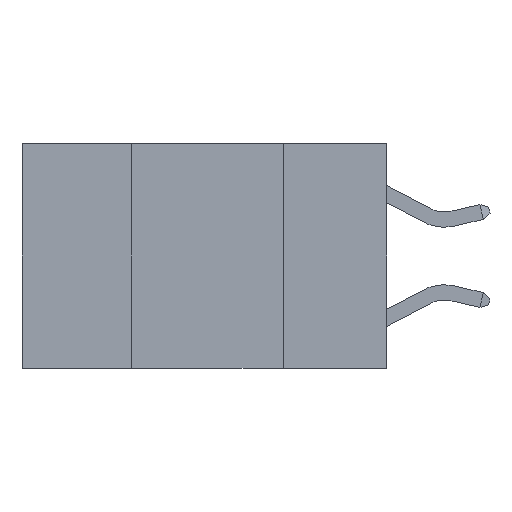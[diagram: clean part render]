
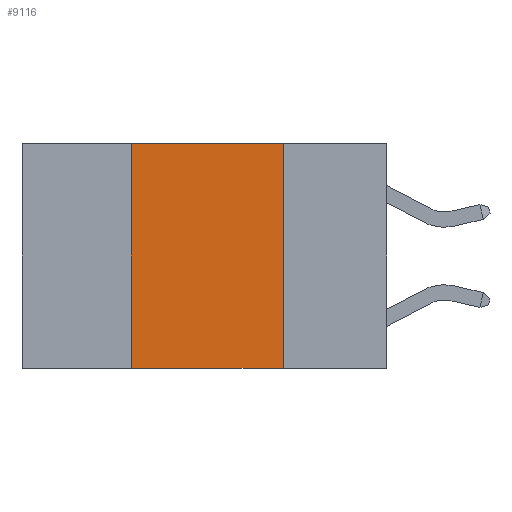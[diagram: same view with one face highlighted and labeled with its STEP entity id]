
A CAD part, left-side view. The second image highlights one B-rep face of the part: STEP entity #9116.
In plain terms, the highlighted planar face has unit normal (-1, 0, 0).
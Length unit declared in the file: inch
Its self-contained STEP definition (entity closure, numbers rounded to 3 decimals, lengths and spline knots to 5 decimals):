
#62 = VECTOR ( 'NONE', #11894, 39.37008 ) ;
#126 = CARTESIAN_POINT ( 'NONE',  ( 0., 0.17, -0.37 ) ) ;
#398 = EDGE_LOOP ( 'NONE', ( #6919, #1309, #10537, #2704 ) ) ;
#486 = VERTEX_POINT ( 'NONE', #126 ) ;
#876 = EDGE_CURVE ( 'NONE', #2681, #11668, #10530, .T. ) ;
#1148 = VECTOR ( 'NONE', #3684, 39.37008 ) ;
#1309 = ORIENTED_EDGE ( 'NONE', *, *, #13399, .F. ) ;
#2628 = LINE ( 'NONE', #9299, #4996 ) ;
#2681 = VERTEX_POINT ( 'NONE', #8434 ) ;
#2704 = ORIENTED_EDGE ( 'NONE', *, *, #11285, .T. ) ;
#3471 = DIRECTION ( 'NONE',  ( 0., 0., -1. ) ) ;
#3684 = DIRECTION ( 'NONE',  ( 0., -1., 0. ) ) ;
#4273 = CARTESIAN_POINT ( 'NONE',  ( 0., 0.17, 0. ) ) ;
#4996 = VECTOR ( 'NONE', #13877, 39.37008 ) ;
#6803 = PLANE ( 'NONE',  #7545 ) ;
#6822 = CARTESIAN_POINT ( 'NONE',  ( 0., 0.42, 0. ) ) ;
#6919 = ORIENTED_EDGE ( 'NONE', *, *, #10854, .F. ) ;
#7545 = AXIS2_PLACEMENT_3D ( 'NONE', #12343, #10077, #3471 ) ;
#7910 = VECTOR ( 'NONE', #11488, 39.37008 ) ;
#8055 = CARTESIAN_POINT ( 'NONE',  ( 0., 0.6, 0. ) ) ;
#8434 = CARTESIAN_POINT ( 'NONE',  ( 0., 0.42, -0.37 ) ) ;
#8445 = CARTESIAN_POINT ( 'NONE',  ( 0., 0.17, 0. ) ) ;
#9116 = ADVANCED_FACE ( 'NONE', ( #13704 ), #6803, .F. ) ;
#9299 = CARTESIAN_POINT ( 'NONE',  ( 0., 0.6, -0.37 ) ) ;
#9623 = VERTEX_POINT ( 'NONE', #4273 ) ;
#9991 = LINE ( 'NONE', #8055, #1148 ) ;
#10077 = DIRECTION ( 'NONE',  ( 1., 0., 0. ) ) ;
#10307 = LINE ( 'NONE', #8445, #62 ) ;
#10530 = LINE ( 'NONE', #12134, #7910 ) ;
#10537 = ORIENTED_EDGE ( 'NONE', *, *, #876, .F. ) ;
#10854 = EDGE_CURVE ( 'NONE', #9623, #486, #10307, .T. ) ;
#11285 = EDGE_CURVE ( 'NONE', #2681, #486, #2628, .T. ) ;
#11488 = DIRECTION ( 'NONE',  ( 0., 0., 1. ) ) ;
#11668 = VERTEX_POINT ( 'NONE', #6822 ) ;
#11894 = DIRECTION ( 'NONE',  ( 0., 0., -1. ) ) ;
#12134 = CARTESIAN_POINT ( 'NONE',  ( 0., 0.42, 0. ) ) ;
#12343 = CARTESIAN_POINT ( 'NONE',  ( 0., 0.6, 0. ) ) ;
#13399 = EDGE_CURVE ( 'NONE', #11668, #9623, #9991, .T. ) ;
#13704 = FACE_OUTER_BOUND ( 'NONE', #398, .T. ) ;
#13877 = DIRECTION ( 'NONE',  ( 0., -1., 0. ) ) ;
